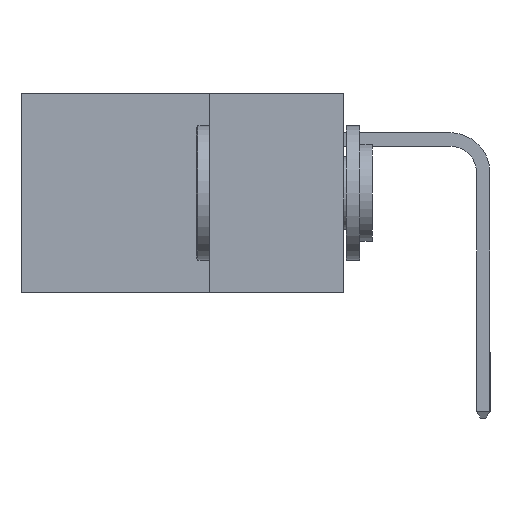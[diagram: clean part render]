
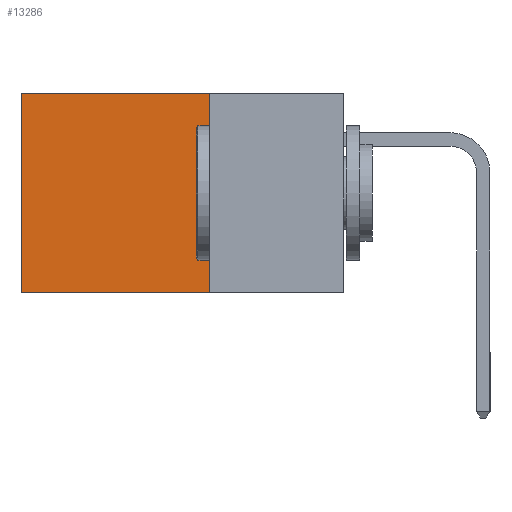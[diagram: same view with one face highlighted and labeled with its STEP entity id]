
A CAD part, left-side view. The second image highlights one B-rep face of the part: STEP entity #13286.
In plain terms, the highlighted planar face has unit normal (-1, 0, 0).
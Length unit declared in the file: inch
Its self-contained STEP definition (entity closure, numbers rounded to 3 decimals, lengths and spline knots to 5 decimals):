
#148 = CARTESIAN_POINT ( 'NONE',  ( 0.298, 0.25, -0.37 ) ) ;
#872 = AXIS2_PLACEMENT_3D ( 'NONE', #3772, #7885, #13375 ) ;
#1532 = CARTESIAN_POINT ( 'NONE',  ( 0.298, 0.6, 0. ) ) ;
#2488 = CARTESIAN_POINT ( 'NONE',  ( 0.298, 0.25, 0. ) ) ;
#3309 = ORIENTED_EDGE ( 'NONE', *, *, #10131, .F. ) ;
#3687 = DIRECTION ( 'NONE',  ( 0., 1., 0. ) ) ;
#3772 = CARTESIAN_POINT ( 'NONE',  ( 0.298, 0.25, 0. ) ) ;
#4592 = CARTESIAN_POINT ( 'NONE',  ( 0.298, 0.25, 0. ) ) ;
#5136 = EDGE_CURVE ( 'NONE', #13591, #11815, #13849, .T. ) ;
#5308 = ORIENTED_EDGE ( 'NONE', *, *, #5136, .T. ) ;
#6666 = VERTEX_POINT ( 'NONE', #9048 ) ;
#7885 = DIRECTION ( 'NONE',  ( 1., 0., 0. ) ) ;
#8486 = LINE ( 'NONE', #13222, #16036 ) ;
#8823 = VECTOR ( 'NONE', #11115, 39.37008 ) ;
#9048 = CARTESIAN_POINT ( 'NONE',  ( 0.298, 0.6, -0.37 ) ) ;
#9088 = ORIENTED_EDGE ( 'NONE', *, *, #11985, .T. ) ;
#9184 = CARTESIAN_POINT ( 'NONE',  ( 0.298, 0.25, -0.37 ) ) ;
#9409 = DIRECTION ( 'NONE',  ( 0., 0., -1. ) ) ;
#10131 = EDGE_CURVE ( 'NONE', #13591, #14581, #8486, .T. ) ;
#10400 = VECTOR ( 'NONE', #16371, 39.37008 ) ;
#11115 = DIRECTION ( 'NONE',  ( 0., 0., -1. ) ) ;
#11815 = VERTEX_POINT ( 'NONE', #17249 ) ;
#11985 = EDGE_CURVE ( 'NONE', #11815, #6666, #16574, .T. ) ;
#12605 = EDGE_CURVE ( 'NONE', #14581, #6666, #15458, .T. ) ;
#12888 = VECTOR ( 'NONE', #3687, 39.37008 ) ;
#13222 = CARTESIAN_POINT ( 'NONE',  ( 0.298, 0.25, 0. ) ) ;
#13286 = ADVANCED_FACE ( 'NONE', ( #14999 ), #14987, .F. ) ;
#13375 = DIRECTION ( 'NONE',  ( 0., 0., -1. ) ) ;
#13591 = VERTEX_POINT ( 'NONE', #4592 ) ;
#13849 = LINE ( 'NONE', #2488, #10400 ) ;
#14581 = VERTEX_POINT ( 'NONE', #148 ) ;
#14987 = PLANE ( 'NONE',  #872 ) ;
#14999 = FACE_OUTER_BOUND ( 'NONE', #15496, .T. ) ;
#15458 = LINE ( 'NONE', #9184, #12888 ) ;
#15496 = EDGE_LOOP ( 'NONE', ( #9088, #17353, #3309, #5308 ) ) ;
#16036 = VECTOR ( 'NONE', #9409, 39.37008 ) ;
#16371 = DIRECTION ( 'NONE',  ( 0., 1., 0. ) ) ;
#16574 = LINE ( 'NONE', #1532, #8823 ) ;
#17249 = CARTESIAN_POINT ( 'NONE',  ( 0.298, 0.6, 0. ) ) ;
#17353 = ORIENTED_EDGE ( 'NONE', *, *, #12605, .F. ) ;
